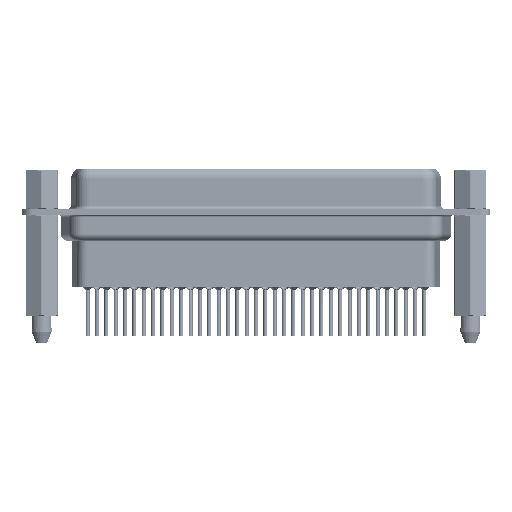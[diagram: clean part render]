
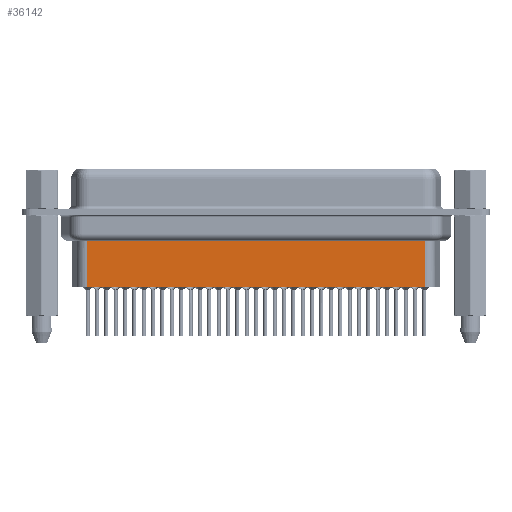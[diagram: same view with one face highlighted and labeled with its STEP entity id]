
A CAD part, front view. The second image highlights one B-rep face of the part: STEP entity #36142.
In plain terms, the highlighted planar face has unit normal (0, -1, 0).
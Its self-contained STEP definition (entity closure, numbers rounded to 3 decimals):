
#616 = CARTESIAN_POINT ( 'NONE',  ( 6.459, -3.5, -4.097 ) ) ;
#4919 = CARTESIAN_POINT ( 'NONE',  ( 6.706, -3.5, -3.1 ) ) ;
#5039 = VERTEX_POINT ( 'NONE', #6337 ) ;
#5707 = LINE ( 'NONE', #4919, #18005 ) ;
#6268 = DIRECTION ( 'NONE',  ( -1., 0., 0. ) ) ;
#6337 = CARTESIAN_POINT ( 'NONE',  ( 56.794, -3.5, -11.15 ) ) ;
#6618 = ORIENTED_EDGE ( 'NONE', *, *, #19596, .T. ) ;
#6852 = VECTOR ( 'NONE', #32915, 1000. ) ;
#8657 = LINE ( 'NONE', #20408, #6852 ) ;
#9323 = EDGE_CURVE ( 'NONE', #5039, #18840, #13292, .T. ) ;
#10108 = FACE_OUTER_BOUND ( 'NONE', #34116, .T. ) ;
#10337 = CARTESIAN_POINT ( 'NONE',  ( 6.706, -3.5, -11.15 ) ) ;
#12741 = LINE ( 'NONE', #616, #16526 ) ;
#13292 = LINE ( 'NONE', #10337, #26263 ) ;
#13942 = DIRECTION ( 'NONE',  ( 0., 0., -1. ) ) ;
#15810 = DIRECTION ( 'NONE',  ( 0., -1., 0. ) ) ;
#16442 = CARTESIAN_POINT ( 'NONE',  ( 6.706, -3.5, -4.097 ) ) ;
#16526 = VECTOR ( 'NONE', #6268, 1000. ) ;
#18005 = VECTOR ( 'NONE', #13942, 1000. ) ;
#18230 = ORIENTED_EDGE ( 'NONE', *, *, #23858, .F. ) ;
#18840 = VERTEX_POINT ( 'NONE', #24564 ) ;
#19528 = DIRECTION ( 'NONE',  ( -1., 0., 0. ) ) ;
#19596 = EDGE_CURVE ( 'NONE', #25728, #18840, #5707, .T. ) ;
#20408 = CARTESIAN_POINT ( 'NONE',  ( 56.794, -3.5, -3.1 ) ) ;
#20602 = ORIENTED_EDGE ( 'NONE', *, *, #37517, .T. ) ;
#21481 = PLANE ( 'NONE',  #30174 ) ;
#21851 = CARTESIAN_POINT ( 'NONE',  ( 6.706, -3.5, -3.1 ) ) ;
#22829 = VERTEX_POINT ( 'NONE', #26508 ) ;
#23858 = EDGE_CURVE ( 'NONE', #22829, #5039, #8657, .T. ) ;
#24564 = CARTESIAN_POINT ( 'NONE',  ( 6.706, -3.5, -11.15 ) ) ;
#25728 = VERTEX_POINT ( 'NONE', #16442 ) ;
#26263 = VECTOR ( 'NONE', #19528, 1000. ) ;
#26508 = CARTESIAN_POINT ( 'NONE',  ( 56.794, -3.5, -4.097 ) ) ;
#30174 = AXIS2_PLACEMENT_3D ( 'NONE', #21851, #15810, #33996 ) ;
#30326 = ORIENTED_EDGE ( 'NONE', *, *, #9323, .F. ) ;
#32915 = DIRECTION ( 'NONE',  ( 0., 0., -1. ) ) ;
#33996 = DIRECTION ( 'NONE',  ( 1., 0., 0. ) ) ;
#34116 = EDGE_LOOP ( 'NONE', ( #18230, #20602, #6618, #30326 ) ) ;
#36142 = ADVANCED_FACE ( 'NONE', ( #10108 ), #21481, .T. ) ;
#37517 = EDGE_CURVE ( 'NONE', #22829, #25728, #12741, .T. ) ;
